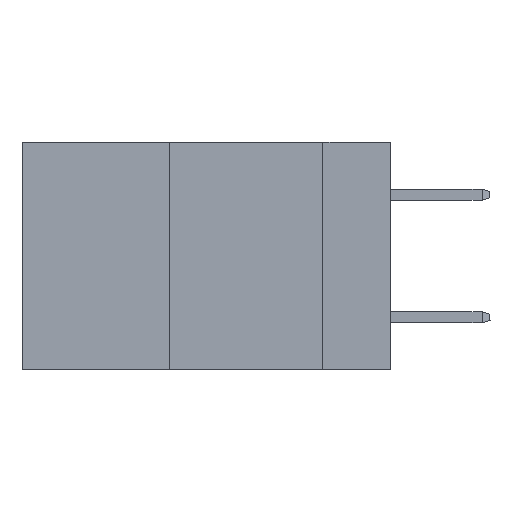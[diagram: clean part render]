
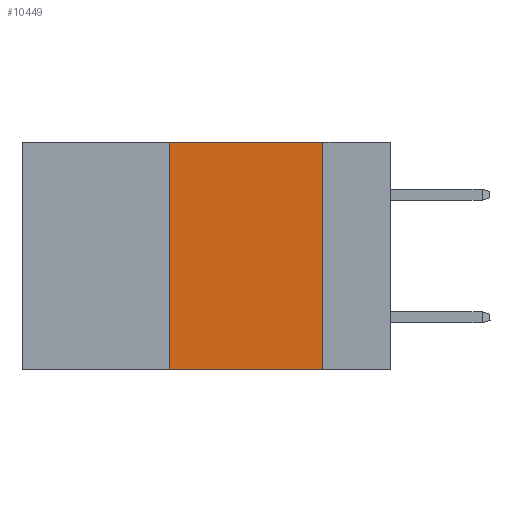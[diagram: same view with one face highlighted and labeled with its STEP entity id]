
A CAD part, left-side view. The second image highlights one B-rep face of the part: STEP entity #10449.
In plain terms, the highlighted planar face has unit normal (-1, 0, 0).
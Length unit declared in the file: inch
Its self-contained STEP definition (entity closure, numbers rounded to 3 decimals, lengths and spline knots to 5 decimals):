
#356 = EDGE_CURVE ( 'NONE', #12364, #21953, #24347, .T. ) ;
#962 = CARTESIAN_POINT ( 'NONE',  ( 0., 0.6, 0. ) ) ;
#1163 = DIRECTION ( 'NONE',  ( 0., -1., 0. ) ) ;
#2157 = CARTESIAN_POINT ( 'NONE',  ( 0., 0.11, -0.37 ) ) ;
#3173 = VECTOR ( 'NONE', #11706, 39.37008 ) ;
#3688 = DIRECTION ( 'NONE',  ( 0., -1., 0. ) ) ;
#4057 = FACE_OUTER_BOUND ( 'NONE', #13856, .T. ) ;
#4833 = ORIENTED_EDGE ( 'NONE', *, *, #9393, .F. ) ;
#6834 = DIRECTION ( 'NONE',  ( 0., 0., -1. ) ) ;
#8134 = VECTOR ( 'NONE', #16744, 39.37008 ) ;
#8878 = LINE ( 'NONE', #25286, #3173 ) ;
#9393 = EDGE_CURVE ( 'NONE', #12364, #19436, #8878, .T. ) ;
#9920 = CARTESIAN_POINT ( 'NONE',  ( 0., 0.36, 0. ) ) ;
#10449 = ADVANCED_FACE ( 'NONE', ( #4057 ), #24661, .F. ) ;
#10499 = CARTESIAN_POINT ( 'NONE',  ( 0., 0.6, -0.37 ) ) ;
#10566 = ORIENTED_EDGE ( 'NONE', *, *, #26737, .F. ) ;
#11706 = DIRECTION ( 'NONE',  ( 0., 0., 1. ) ) ;
#12364 = VERTEX_POINT ( 'NONE', #19544 ) ;
#13271 = AXIS2_PLACEMENT_3D ( 'NONE', #24760, #18352, #6834 ) ;
#13605 = VECTOR ( 'NONE', #1163, 39.37008 ) ;
#13856 = EDGE_LOOP ( 'NONE', ( #25061, #10566, #4833, #19033 ) ) ;
#14771 = VERTEX_POINT ( 'NONE', #22143 ) ;
#15998 = LINE ( 'NONE', #962, #13605 ) ;
#16647 = CARTESIAN_POINT ( 'NONE',  ( 0., 0.11, 0. ) ) ;
#16744 = DIRECTION ( 'NONE',  ( 0., 0., -1. ) ) ;
#17395 = EDGE_CURVE ( 'NONE', #14771, #21953, #17985, .T. ) ;
#17985 = LINE ( 'NONE', #16647, #8134 ) ;
#18352 = DIRECTION ( 'NONE',  ( 1., 0., 0. ) ) ;
#19033 = ORIENTED_EDGE ( 'NONE', *, *, #356, .T. ) ;
#19436 = VERTEX_POINT ( 'NONE', #9920 ) ;
#19544 = CARTESIAN_POINT ( 'NONE',  ( 0., 0.36, -0.37 ) ) ;
#21953 = VERTEX_POINT ( 'NONE', #2157 ) ;
#22143 = CARTESIAN_POINT ( 'NONE',  ( 0., 0.11, 0. ) ) ;
#24347 = LINE ( 'NONE', #10499, #27867 ) ;
#24661 = PLANE ( 'NONE',  #13271 ) ;
#24760 = CARTESIAN_POINT ( 'NONE',  ( 0., 0.6, 0. ) ) ;
#25061 = ORIENTED_EDGE ( 'NONE', *, *, #17395, .F. ) ;
#25286 = CARTESIAN_POINT ( 'NONE',  ( 0., 0.36, 0. ) ) ;
#26737 = EDGE_CURVE ( 'NONE', #19436, #14771, #15998, .T. ) ;
#27867 = VECTOR ( 'NONE', #3688, 39.37008 ) ;
